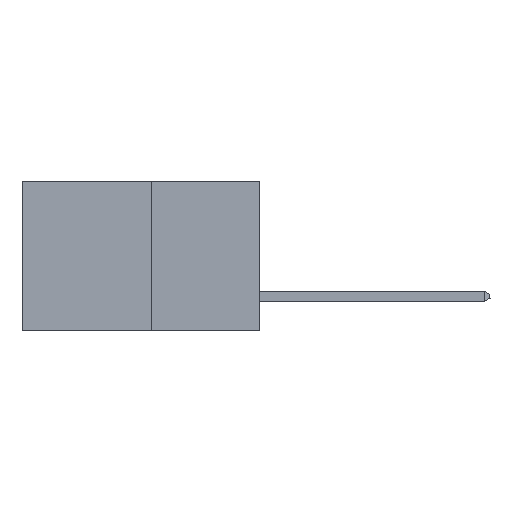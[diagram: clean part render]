
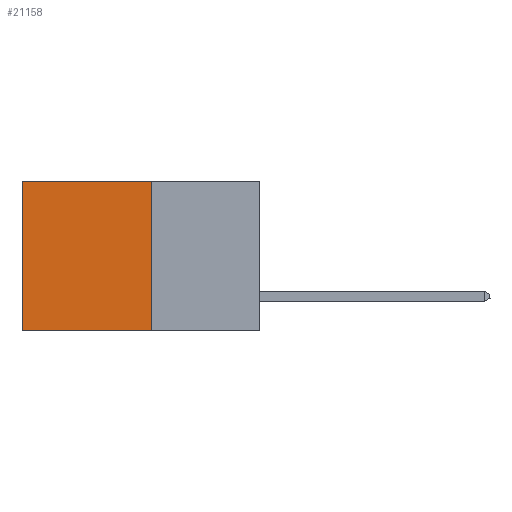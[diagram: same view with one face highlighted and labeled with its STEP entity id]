
A CAD part, left-side view. The second image highlights one B-rep face of the part: STEP entity #21158.
In plain terms, the highlighted planar face has unit normal (-1, 0, 0).
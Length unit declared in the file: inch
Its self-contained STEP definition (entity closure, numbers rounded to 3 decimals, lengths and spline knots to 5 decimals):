
#200 = VECTOR ( 'NONE', #28553, 39.37008 ) ;
#1059 = VERTEX_POINT ( 'NONE', #16879 ) ;
#1420 = EDGE_LOOP ( 'NONE', ( #21987, #8378, #15773, #12142 ) ) ;
#3494 = VERTEX_POINT ( 'NONE', #26258 ) ;
#3812 = VECTOR ( 'NONE', #22398, 39.37008 ) ;
#4312 = CARTESIAN_POINT ( 'NONE',  ( 0.277, 0.59, -0.37 ) ) ;
#5635 = FACE_OUTER_BOUND ( 'NONE', #1420, .T. ) ;
#7570 = EDGE_CURVE ( 'NONE', #17806, #3494, #20297, .T. ) ;
#8378 = ORIENTED_EDGE ( 'NONE', *, *, #17083, .F. ) ;
#8440 = PLANE ( 'NONE',  #29059 ) ;
#11032 = DIRECTION ( 'NONE',  ( 0., 0., -1. ) ) ;
#12142 = ORIENTED_EDGE ( 'NONE', *, *, #7570, .T. ) ;
#15773 = ORIENTED_EDGE ( 'NONE', *, *, #26400, .F. ) ;
#16111 = CARTESIAN_POINT ( 'NONE',  ( 0.277, 0.27, -0.37 ) ) ;
#16879 = CARTESIAN_POINT ( 'NONE',  ( 0.277, 0.59, -0.37 ) ) ;
#17083 = EDGE_CURVE ( 'NONE', #31341, #1059, #29309, .T. ) ;
#17806 = VERTEX_POINT ( 'NONE', #19612 ) ;
#18226 = CARTESIAN_POINT ( 'NONE',  ( 0.277, 0.27, -0.37 ) ) ;
#19333 = CARTESIAN_POINT ( 'NONE',  ( 0.277, 0.27, 0. ) ) ;
#19612 = CARTESIAN_POINT ( 'NONE',  ( 0.277, 0.27, 0. ) ) ;
#20297 = LINE ( 'NONE', #19333, #33122 ) ;
#21158 = ADVANCED_FACE ( 'NONE', ( #5635 ), #8440, .F. ) ;
#21909 = DIRECTION ( 'NONE',  ( 0., 1., 0. ) ) ;
#21987 = ORIENTED_EDGE ( 'NONE', *, *, #23371, .T. ) ;
#22398 = DIRECTION ( 'NONE',  ( 0., 0., -1. ) ) ;
#22449 = DIRECTION ( 'NONE',  ( 0., 1., 0. ) ) ;
#22475 = VECTOR ( 'NONE', #22449, 39.37008 ) ;
#22849 = LINE ( 'NONE', #4312, #3812 ) ;
#23371 = EDGE_CURVE ( 'NONE', #3494, #1059, #22849, .T. ) ;
#26258 = CARTESIAN_POINT ( 'NONE',  ( 0.277, 0.59, 0. ) ) ;
#26400 = EDGE_CURVE ( 'NONE', #17806, #31341, #27795, .T. ) ;
#26456 = DIRECTION ( 'NONE',  ( 1., 0., 0. ) ) ;
#27795 = LINE ( 'NONE', #18226, #200 ) ;
#28553 = DIRECTION ( 'NONE',  ( 0., 0., -1. ) ) ;
#29059 = AXIS2_PLACEMENT_3D ( 'NONE', #16111, #26456, #11032 ) ;
#29309 = LINE ( 'NONE', #32652, #22475 ) ;
#29397 = CARTESIAN_POINT ( 'NONE',  ( 0.277, 0.27, -0.37 ) ) ;
#31341 = VERTEX_POINT ( 'NONE', #29397 ) ;
#32652 = CARTESIAN_POINT ( 'NONE',  ( 0.277, 0.27, -0.37 ) ) ;
#33122 = VECTOR ( 'NONE', #21909, 39.37008 ) ;
